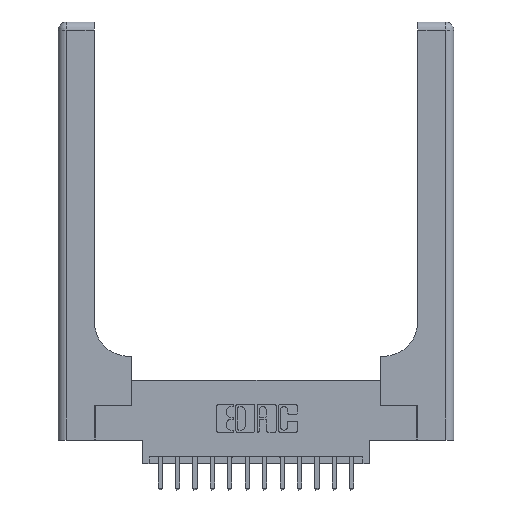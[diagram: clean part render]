
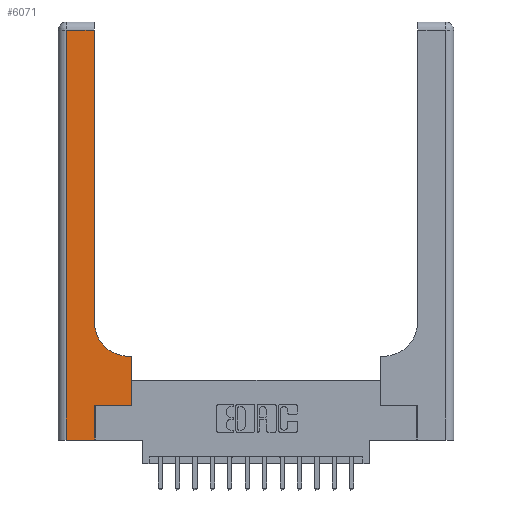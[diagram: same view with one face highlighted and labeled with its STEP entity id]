
A CAD part, top view. The second image highlights one B-rep face of the part: STEP entity #6071.
In plain terms, the highlighted planar face has unit normal (0, 0, 1).
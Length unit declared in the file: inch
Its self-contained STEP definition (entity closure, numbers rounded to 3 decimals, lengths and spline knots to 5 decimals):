
#101 = ORIENTED_EDGE ( 'NONE', *, *, #4524, .T. ) ;
#674 = DIRECTION ( 'NONE',  ( 0., 1., 0. ) ) ;
#713 = EDGE_CURVE ( 'NONE', #884, #2022, #17103, .T. ) ;
#884 = VERTEX_POINT ( 'NONE', #7873 ) ;
#894 = EDGE_CURVE ( 'NONE', #1097, #1183, #7820, .T. ) ;
#1011 = CARTESIAN_POINT ( 'NONE',  ( 0.528, 0.25, 0.37 ) ) ;
#1097 = VERTEX_POINT ( 'NONE', #3475 ) ;
#1183 = VERTEX_POINT ( 'NONE', #1011 ) ;
#1194 = CARTESIAN_POINT ( 'NONE',  ( 0.26, 0.6, 0.37 ) ) ;
#2022 = VERTEX_POINT ( 'NONE', #15349 ) ;
#2262 = EDGE_CURVE ( 'NONE', #9244, #11139, #7385, .T. ) ;
#2960 = ORIENTED_EDGE ( 'NONE', *, *, #3644, .T. ) ;
#3475 = CARTESIAN_POINT ( 'NONE',  ( 0.265, 0.25, 0.37 ) ) ;
#3644 = EDGE_CURVE ( 'NONE', #11139, #8578, #13230, .T. ) ;
#3755 = VECTOR ( 'NONE', #9570, 39.37008 ) ;
#3880 = EDGE_CURVE ( 'NONE', #8578, #1097, #10798, .T. ) ;
#4025 = CARTESIAN_POINT ( 'NONE',  ( 0.528, 0.6, 0.37 ) ) ;
#4187 = VECTOR ( 'NONE', #7726, 39.37008 ) ;
#4333 = VECTOR ( 'NONE', #9991, 39.37008 ) ;
#4524 = EDGE_CURVE ( 'NONE', #16044, #9244, #11389, .T. ) ;
#4579 = CARTESIAN_POINT ( 'NONE',  ( 0.265, 0., 0.37 ) ) ;
#4644 = ORIENTED_EDGE ( 'NONE', *, *, #3880, .T. ) ;
#4767 = DIRECTION ( 'NONE',  ( 0., 1., 0. ) ) ;
#4782 = CARTESIAN_POINT ( 'NONE',  ( 0.528, 0.25, 0.37 ) ) ;
#5687 = LINE ( 'NONE', #14179, #12682 ) ;
#5835 = ORIENTED_EDGE ( 'NONE', *, *, #16717, .T. ) ;
#6004 = DIRECTION ( 'NONE',  ( -1., 0., 0. ) ) ;
#6009 = DIRECTION ( 'NONE',  ( 0., 0., -1. ) ) ;
#6031 = PLANE ( 'NONE',  #15908 ) ;
#6071 = ADVANCED_FACE ( 'NONE', ( #11776 ), #6031, .F. ) ;
#6140 = CARTESIAN_POINT ( 'NONE',  ( 0., 3., 0.37 ) ) ;
#6165 = EDGE_LOOP ( 'NONE', ( #5835, #101, #9058, #2960, #4644, #9804, #15244, #17066, #10626 ) ) ;
#6361 = DIRECTION ( 'NONE',  ( 0., 1., 0. ) ) ;
#6728 = DIRECTION ( 'NONE',  ( -1., 0., 0. ) ) ;
#6852 = AXIS2_PLACEMENT_3D ( 'NONE', #10948, #10929, #10913 ) ;
#7106 = VECTOR ( 'NONE', #674, 39.37008 ) ;
#7385 = LINE ( 'NONE', #9546, #3755 ) ;
#7647 = DIRECTION ( 'NONE',  ( 1., 0., 0. ) ) ;
#7726 = DIRECTION ( 'NONE',  ( 1., 0., 0. ) ) ;
#7820 = LINE ( 'NONE', #8210, #4187 ) ;
#7873 = CARTESIAN_POINT ( 'NONE',  ( 0.51, 0.6, 0.37 ) ) ;
#8145 = CARTESIAN_POINT ( 'NONE',  ( 0., 0., 0.37 ) ) ;
#8210 = CARTESIAN_POINT ( 'NONE',  ( 0.265, 0.25, 0.37 ) ) ;
#8578 = VERTEX_POINT ( 'NONE', #13862 ) ;
#9058 = ORIENTED_EDGE ( 'NONE', *, *, #2262, .T. ) ;
#9186 = VERTEX_POINT ( 'NONE', #4025 ) ;
#9244 = VERTEX_POINT ( 'NONE', #17272 ) ;
#9546 = CARTESIAN_POINT ( 'NONE',  ( 0.06, 3., 0.37 ) ) ;
#9570 = DIRECTION ( 'NONE',  ( 0., -1., 0. ) ) ;
#9804 = ORIENTED_EDGE ( 'NONE', *, *, #894, .T. ) ;
#9991 = DIRECTION ( 'NONE',  ( -1., 0., 0. ) ) ;
#9996 = VECTOR ( 'NONE', #4767, 39.37008 ) ;
#10008 = CARTESIAN_POINT ( 'NONE',  ( 0., 2.94, 0.37 ) ) ;
#10094 = LINE ( 'NONE', #1194, #13516 ) ;
#10626 = ORIENTED_EDGE ( 'NONE', *, *, #713, .T. ) ;
#10798 = LINE ( 'NONE', #4579, #9996 ) ;
#10913 = DIRECTION ( 'NONE',  ( 1., 0., 0. ) ) ;
#10929 = DIRECTION ( 'NONE',  ( 0., 0., -1. ) ) ;
#10948 = CARTESIAN_POINT ( 'NONE',  ( 0.51, 0.85, 0.37 ) ) ;
#11139 = VERTEX_POINT ( 'NONE', #15112 ) ;
#11194 = EDGE_CURVE ( 'NONE', #1183, #9186, #13212, .T. ) ;
#11389 = LINE ( 'NONE', #10008, #4333 ) ;
#11776 = FACE_OUTER_BOUND ( 'NONE', #6165, .T. ) ;
#12682 = VECTOR ( 'NONE', #6361, 39.37008 ) ;
#12804 = CARTESIAN_POINT ( 'NONE',  ( 0.26, 2.94, 0.37 ) ) ;
#12839 = VECTOR ( 'NONE', #7647, 39.37008 ) ;
#13212 = LINE ( 'NONE', #4782, #7106 ) ;
#13230 = LINE ( 'NONE', #8145, #12839 ) ;
#13516 = VECTOR ( 'NONE', #6728, 39.37008 ) ;
#13862 = CARTESIAN_POINT ( 'NONE',  ( 0.265, 0., 0.37 ) ) ;
#14179 = CARTESIAN_POINT ( 'NONE',  ( 0.26, 3., 0.37 ) ) ;
#14559 = EDGE_CURVE ( 'NONE', #9186, #884, #10094, .T. ) ;
#15112 = CARTESIAN_POINT ( 'NONE',  ( 0.06, 0., 0.37 ) ) ;
#15244 = ORIENTED_EDGE ( 'NONE', *, *, #11194, .T. ) ;
#15349 = CARTESIAN_POINT ( 'NONE',  ( 0.26, 0.85, 0.37 ) ) ;
#15908 = AXIS2_PLACEMENT_3D ( 'NONE', #6140, #6009, #6004 ) ;
#16044 = VERTEX_POINT ( 'NONE', #12804 ) ;
#16717 = EDGE_CURVE ( 'NONE', #2022, #16044, #5687, .T. ) ;
#17066 = ORIENTED_EDGE ( 'NONE', *, *, #14559, .T. ) ;
#17103 = CIRCLE ( 'NONE', #6852, 0.25 ) ;
#17272 = CARTESIAN_POINT ( 'NONE',  ( 0.06, 2.94, 0.37 ) ) ;
